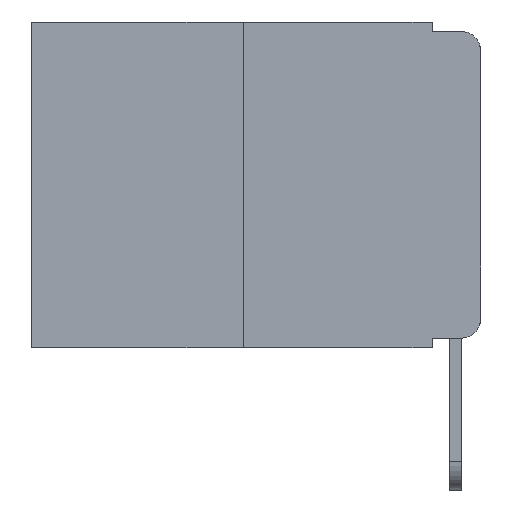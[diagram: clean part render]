
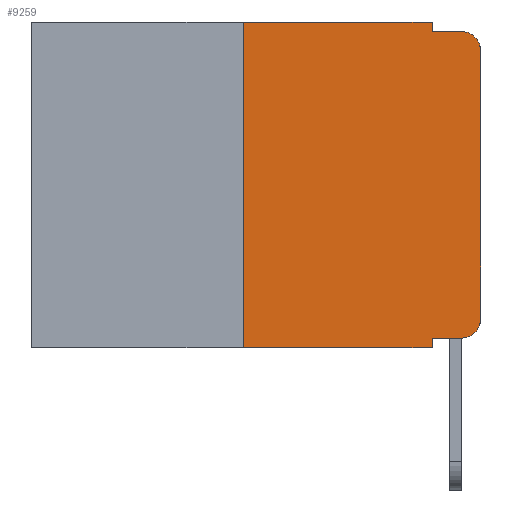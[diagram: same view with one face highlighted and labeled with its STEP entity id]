
A CAD part, left-side view. The second image highlights one B-rep face of the part: STEP entity #9259.
In plain terms, the highlighted planar face has unit normal (-1, 0, 0).
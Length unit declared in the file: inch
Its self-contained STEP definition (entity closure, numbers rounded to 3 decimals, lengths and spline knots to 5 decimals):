
#9 = ORIENTED_EDGE ( 'NONE', *, *, #7236, .T. ) ;
#103 = VERTEX_POINT ( 'NONE', #10662 ) ;
#170 = CARTESIAN_POINT ( 'NONE',  ( 0., 0.051, -0.343 ) ) ;
#280 = CARTESIAN_POINT ( 'NONE',  ( 0., 0.25, 0. ) ) ;
#755 = VERTEX_POINT ( 'NONE', #10330 ) ;
#845 = AXIS2_PLACEMENT_3D ( 'NONE', #1557, #10720, #4573 ) ;
#932 = ORIENTED_EDGE ( 'NONE', *, *, #4374, .T. ) ;
#1102 = ORIENTED_EDGE ( 'NONE', *, *, #5349, .T. ) ;
#1502 = EDGE_LOOP ( 'NONE', ( #932, #1102, #1555, #1953, #2860, #3484, #4718, #9530, #9, #1534 ) ) ;
#1505 = VERTEX_POINT ( 'NONE', #280 ) ;
#1534 = ORIENTED_EDGE ( 'NONE', *, *, #2495, .T. ) ;
#1543 = CARTESIAN_POINT ( 'NONE',  ( 0., 0.051, -0.01 ) ) ;
#1555 = ORIENTED_EDGE ( 'NONE', *, *, #5632, .F. ) ;
#1557 = CARTESIAN_POINT ( 'NONE',  ( 0., 0.473, 0. ) ) ;
#1567 = AXIS2_PLACEMENT_3D ( 'NONE', #10665, #13179, #2107 ) ;
#1599 = LINE ( 'NONE', #12845, #11979 ) ;
#1640 = VERTEX_POINT ( 'NONE', #9493 ) ;
#1953 = ORIENTED_EDGE ( 'NONE', *, *, #5991, .F. ) ;
#2107 = DIRECTION ( 'NONE',  ( 0., 0., -1. ) ) ;
#2227 = LINE ( 'NONE', #11312, #4221 ) ;
#2495 = EDGE_CURVE ( 'NONE', #4182, #3577, #5176, .T. ) ;
#2547 = VECTOR ( 'NONE', #10677, 39.37008 ) ;
#2595 = CARTESIAN_POINT ( 'NONE',  ( 0., 0.25, -0.343 ) ) ;
#2738 = LINE ( 'NONE', #13152, #10215 ) ;
#2860 = ORIENTED_EDGE ( 'NONE', *, *, #7924, .F. ) ;
#2893 = CARTESIAN_POINT ( 'NONE',  ( 0., 0.02, -0.01 ) ) ;
#2938 = VERTEX_POINT ( 'NONE', #2893 ) ;
#3062 = EDGE_CURVE ( 'NONE', #8057, #4482, #10334, .T. ) ;
#3080 = DIRECTION ( 'NONE',  ( 0., 0., 1. ) ) ;
#3277 = VECTOR ( 'NONE', #5639, 39.37008 ) ;
#3484 = ORIENTED_EDGE ( 'NONE', *, *, #6008, .F. ) ;
#3577 = VERTEX_POINT ( 'NONE', #10691 ) ;
#4182 = VERTEX_POINT ( 'NONE', #9062 ) ;
#4221 = VECTOR ( 'NONE', #8304, 39.37008 ) ;
#4374 = EDGE_CURVE ( 'NONE', #3577, #755, #12481, .T. ) ;
#4482 = VERTEX_POINT ( 'NONE', #170 ) ;
#4541 = PLANE ( 'NONE',  #845 ) ;
#4573 = DIRECTION ( 'NONE',  ( 0., 0., -1. ) ) ;
#4718 = ORIENTED_EDGE ( 'NONE', *, *, #3062, .T. ) ;
#5176 = CIRCLE ( 'NONE', #10772, 0.02 ) ;
#5237 = DIRECTION ( 'NONE',  ( 0., -1., 0. ) ) ;
#5349 = EDGE_CURVE ( 'NONE', #755, #2938, #11472, .T. ) ;
#5632 = EDGE_CURVE ( 'NONE', #1640, #2938, #8661, .T. ) ;
#5639 = DIRECTION ( 'NONE',  ( 0., -1., 0. ) ) ;
#5962 = VECTOR ( 'NONE', #11487, 39.37008 ) ;
#5991 = EDGE_CURVE ( 'NONE', #10851, #1640, #1599, .T. ) ;
#6008 = EDGE_CURVE ( 'NONE', #8057, #1505, #9457, .T. ) ;
#6123 = CARTESIAN_POINT ( 'NONE',  ( 0., 0., 0. ) ) ;
#6262 = DIRECTION ( 'NONE',  ( 0., 0., 1. ) ) ;
#6300 = CARTESIAN_POINT ( 'NONE',  ( 0., 0.25, 0. ) ) ;
#6567 = DIRECTION ( 'NONE',  ( 0., 0., -1. ) ) ;
#7146 = EDGE_CURVE ( 'NONE', #103, #4482, #11962, .T. ) ;
#7154 = VECTOR ( 'NONE', #6262, 39.37008 ) ;
#7236 = EDGE_CURVE ( 'NONE', #103, #4182, #2738, .T. ) ;
#7924 = EDGE_CURVE ( 'NONE', #1505, #10851, #2227, .T. ) ;
#8057 = VERTEX_POINT ( 'NONE', #2595 ) ;
#8304 = DIRECTION ( 'NONE',  ( 0., -1., 0. ) ) ;
#8661 = LINE ( 'NONE', #1543, #3277 ) ;
#9062 = CARTESIAN_POINT ( 'NONE',  ( 0., 0.02, -0.333 ) ) ;
#9156 = CARTESIAN_POINT ( 'NONE',  ( 0., 0.051, 0. ) ) ;
#9259 = ADVANCED_FACE ( 'NONE', ( #10703 ), #4541, .F. ) ;
#9457 = LINE ( 'NONE', #6300, #11711 ) ;
#9493 = CARTESIAN_POINT ( 'NONE',  ( 0., 0.051, -0.01 ) ) ;
#9530 = ORIENTED_EDGE ( 'NONE', *, *, #7146, .F. ) ;
#10215 = VECTOR ( 'NONE', #5237, 39.37008 ) ;
#10262 = CARTESIAN_POINT ( 'NONE',  ( 0., 0.051, 0. ) ) ;
#10330 = CARTESIAN_POINT ( 'NONE',  ( 0., 0., -0.03 ) ) ;
#10334 = LINE ( 'NONE', #12597, #2547 ) ;
#10662 = CARTESIAN_POINT ( 'NONE',  ( 0., 0.051, -0.333 ) ) ;
#10665 = CARTESIAN_POINT ( 'NONE',  ( 0., 0.02, -0.03 ) ) ;
#10677 = DIRECTION ( 'NONE',  ( 0., -1., 0. ) ) ;
#10691 = CARTESIAN_POINT ( 'NONE',  ( 0., 0., -0.313 ) ) ;
#10703 = FACE_OUTER_BOUND ( 'NONE', #1502, .T. ) ;
#10720 = DIRECTION ( 'NONE',  ( 1., 0., 0. ) ) ;
#10772 = AXIS2_PLACEMENT_3D ( 'NONE', #11219, #11135, #11126 ) ;
#10851 = VERTEX_POINT ( 'NONE', #10262 ) ;
#11126 = DIRECTION ( 'NONE',  ( 0., 0., -1. ) ) ;
#11135 = DIRECTION ( 'NONE',  ( -1., 0., 0. ) ) ;
#11219 = CARTESIAN_POINT ( 'NONE',  ( 0., 0.02, -0.313 ) ) ;
#11312 = CARTESIAN_POINT ( 'NONE',  ( 0., 0.473, 0. ) ) ;
#11472 = CIRCLE ( 'NONE', #1567, 0.02 ) ;
#11487 = DIRECTION ( 'NONE',  ( 0., 0., -1. ) ) ;
#11711 = VECTOR ( 'NONE', #3080, 39.37008 ) ;
#11962 = LINE ( 'NONE', #9156, #5962 ) ;
#11979 = VECTOR ( 'NONE', #6567, 39.37008 ) ;
#12481 = LINE ( 'NONE', #6123, #7154 ) ;
#12597 = CARTESIAN_POINT ( 'NONE',  ( 0., 0.473, -0.343 ) ) ;
#12845 = CARTESIAN_POINT ( 'NONE',  ( 0., 0.051, 0. ) ) ;
#13152 = CARTESIAN_POINT ( 'NONE',  ( 0., 0.051, -0.333 ) ) ;
#13179 = DIRECTION ( 'NONE',  ( -1., 0., 0. ) ) ;
